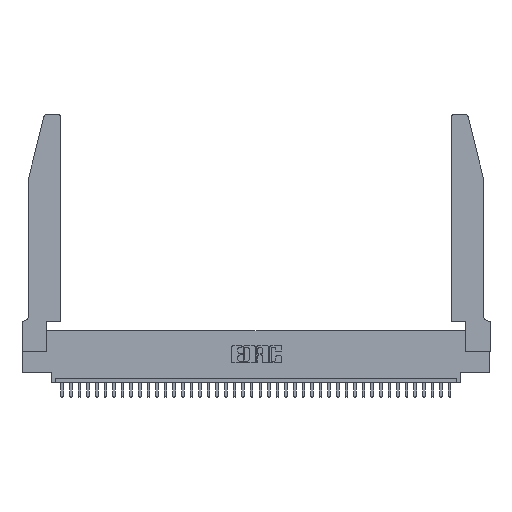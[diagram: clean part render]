
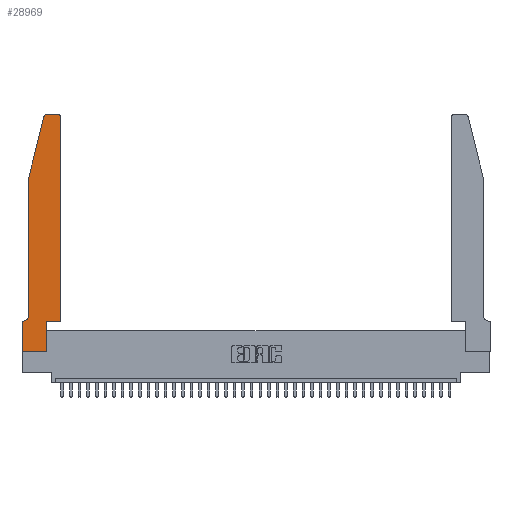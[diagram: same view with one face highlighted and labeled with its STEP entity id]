
A CAD part, top view. The second image highlights one B-rep face of the part: STEP entity #28969.
In plain terms, the highlighted planar face has unit normal (0, 0, 1).
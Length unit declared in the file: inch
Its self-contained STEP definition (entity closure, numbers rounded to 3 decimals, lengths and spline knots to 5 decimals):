
#128 = LINE ( 'NONE', #25591, #30312 ) ;
#791 = CARTESIAN_POINT ( 'NONE',  ( 0.4505, 0.35, 0.37 ) ) ;
#982 = CARTESIAN_POINT ( 'NONE',  ( 0.4505, 0.35, 0.37 ) ) ;
#1350 = VECTOR ( 'NONE', #25044, 39.37008 ) ;
#1521 = VERTEX_POINT ( 'NONE', #6989 ) ;
#1941 = CARTESIAN_POINT ( 'NONE',  ( 0., 0.35, 0.37 ) ) ;
#2319 = LINE ( 'NONE', #22248, #1350 ) ;
#2846 = EDGE_CURVE ( 'NONE', #31651, #19079, #12130, .T. ) ;
#3792 = DIRECTION ( 'NONE',  ( -1., 0., 0. ) ) ;
#3812 = DIRECTION ( 'NONE',  ( 1., 0., 0. ) ) ;
#4138 = DIRECTION ( 'NONE',  ( 0., 0., 1. ) ) ;
#4660 = DIRECTION ( 'NONE',  ( 1., 0., 0. ) ) ;
#4921 = ORIENTED_EDGE ( 'NONE', *, *, #25718, .T. ) ;
#4977 = VERTEX_POINT ( 'NONE', #23273 ) ;
#5688 = VECTOR ( 'NONE', #35818, 39.37008 ) ;
#5738 = VERTEX_POINT ( 'NONE', #27269 ) ;
#5854 = DIRECTION ( 'NONE',  ( 0., -1., 0. ) ) ;
#6151 = EDGE_CURVE ( 'NONE', #10731, #8909, #2319, .T. ) ;
#6451 = VERTEX_POINT ( 'NONE', #10563 ) ;
#6634 = ORIENTED_EDGE ( 'NONE', *, *, #23860, .T. ) ;
#6649 = LINE ( 'NONE', #34305, #27004 ) ;
#6671 = EDGE_LOOP ( 'NONE', ( #28774, #6634, #18262, #8456, #10454, #37717, #17389, #11068, #31452, #4921, #36586, #11282 ) ) ;
#6717 = VECTOR ( 'NONE', #5854, 39.37008 ) ;
#6989 = CARTESIAN_POINT ( 'NONE',  ( 0.2865, 0., 0.37 ) ) ;
#7357 = VERTEX_POINT ( 'NONE', #791 ) ;
#7821 = AXIS2_PLACEMENT_3D ( 'NONE', #34292, #33864, #3812 ) ;
#7995 = PLANE ( 'NONE',  #35997 ) ;
#8456 = ORIENTED_EDGE ( 'NONE', *, *, #28967, .T. ) ;
#8909 = VERTEX_POINT ( 'NONE', #16999 ) ;
#9334 = CARTESIAN_POINT ( 'NONE',  ( 0.2865, 0.35, 0.37 ) ) ;
#9813 = DIRECTION ( 'NONE',  ( 0., 0., -1. ) ) ;
#10454 = ORIENTED_EDGE ( 'NONE', *, *, #38095, .T. ) ;
#10563 = CARTESIAN_POINT ( 'NONE',  ( 0.25487, 2.72718, 0.37 ) ) ;
#10731 = VERTEX_POINT ( 'NONE', #34325 ) ;
#11068 = ORIENTED_EDGE ( 'NONE', *, *, #13427, .T. ) ;
#11282 = ORIENTED_EDGE ( 'NONE', *, *, #33026, .T. ) ;
#11543 = DIRECTION ( 'NONE',  ( 1., 0., 0. ) ) ;
#11690 = CARTESIAN_POINT ( 'NONE',  ( 0.0755, 2., 0.37 ) ) ;
#11742 = LINE ( 'NONE', #982, #18739 ) ;
#11847 = LINE ( 'NONE', #9334, #31189 ) ;
#12130 = LINE ( 'NONE', #37443, #17319 ) ;
#13427 = EDGE_CURVE ( 'NONE', #4977, #1521, #6649, .T. ) ;
#14121 = EDGE_CURVE ( 'NONE', #1521, #28486, #11847, .T. ) ;
#14594 = FACE_OUTER_BOUND ( 'NONE', #6671, .T. ) ;
#15900 = DIRECTION ( 'NONE',  ( -1., 0., 0. ) ) ;
#15913 = EDGE_CURVE ( 'NONE', #7357, #5738, #11742, .T. ) ;
#16732 = DIRECTION ( 'NONE',  ( 1., 0., 0. ) ) ;
#16999 = CARTESIAN_POINT ( 'NONE',  ( 0., 0.35, 0.37 ) ) ;
#17319 = VECTOR ( 'NONE', #3792, 39.37008 ) ;
#17389 = ORIENTED_EDGE ( 'NONE', *, *, #32814, .T. ) ;
#17987 = CIRCLE ( 'NONE', #26717, 0.03 ) ;
#18262 = ORIENTED_EDGE ( 'NONE', *, *, #22320, .T. ) ;
#18739 = VECTOR ( 'NONE', #24847, 39.37008 ) ;
#19079 = VERTEX_POINT ( 'NONE', #31650 ) ;
#19757 = AXIS2_PLACEMENT_3D ( 'NONE', #37557, #9813, #15900 ) ;
#19985 = DIRECTION ( 'NONE',  ( 0., -1., 0. ) ) ;
#21511 = CARTESIAN_POINT ( 'NONE',  ( 0., 0., 0.37 ) ) ;
#22248 = CARTESIAN_POINT ( 'NONE',  ( 0.0755, 0.35, 0.37 ) ) ;
#22320 = EDGE_CURVE ( 'NONE', #6451, #22796, #26927, .T. ) ;
#22796 = VERTEX_POINT ( 'NONE', #31277 ) ;
#23273 = CARTESIAN_POINT ( 'NONE',  ( 0., 0., 0.37 ) ) ;
#23291 = LINE ( 'NONE', #21511, #6717 ) ;
#23860 = EDGE_CURVE ( 'NONE', #19079, #6451, #23974, .T. ) ;
#23974 = CIRCLE ( 'NONE', #7821, 0.03 ) ;
#24756 = CARTESIAN_POINT ( 'NONE',  ( 0.2865, 0.35, 0.37 ) ) ;
#24847 = DIRECTION ( 'NONE',  ( 0., 1., 0. ) ) ;
#25044 = DIRECTION ( 'NONE',  ( -1., 0., 0. ) ) ;
#25152 = VERTEX_POINT ( 'NONE', #37725 ) ;
#25591 = CARTESIAN_POINT ( 'NONE',  ( 0.4505, 0.35, 0.37 ) ) ;
#25718 = EDGE_CURVE ( 'NONE', #28486, #7357, #128, .T. ) ;
#26717 = AXIS2_PLACEMENT_3D ( 'NONE', #37647, #4138, #37366 ) ;
#26855 = LINE ( 'NONE', #34243, #36708 ) ;
#26927 = LINE ( 'NONE', #11690, #5688 ) ;
#27004 = VECTOR ( 'NONE', #4660, 39.37008 ) ;
#27269 = CARTESIAN_POINT ( 'NONE',  ( 0.4505, 2.72, 0.37 ) ) ;
#28486 = VERTEX_POINT ( 'NONE', #24756 ) ;
#28774 = ORIENTED_EDGE ( 'NONE', *, *, #2846, .T. ) ;
#28967 = EDGE_CURVE ( 'NONE', #22796, #25152, #26855, .T. ) ;
#28969 = ADVANCED_FACE ( 'NONE', ( #14594 ), #7995, .T. ) ;
#29035 = CIRCLE ( 'NONE', #19757, 0.07 ) ;
#30312 = VECTOR ( 'NONE', #16732, 39.37008 ) ;
#31137 = DIRECTION ( 'NONE',  ( 0., 1., 0. ) ) ;
#31189 = VECTOR ( 'NONE', #31137, 39.37008 ) ;
#31277 = CARTESIAN_POINT ( 'NONE',  ( 0.0755, 2., 0.37 ) ) ;
#31452 = ORIENTED_EDGE ( 'NONE', *, *, #14121, .T. ) ;
#31650 = CARTESIAN_POINT ( 'NONE',  ( 0.284, 2.75, 0.37 ) ) ;
#31651 = VERTEX_POINT ( 'NONE', #36376 ) ;
#32814 = EDGE_CURVE ( 'NONE', #8909, #4977, #23291, .T. ) ;
#33026 = EDGE_CURVE ( 'NONE', #5738, #31651, #17987, .T. ) ;
#33864 = DIRECTION ( 'NONE',  ( 0., 0., 1. ) ) ;
#34243 = CARTESIAN_POINT ( 'NONE',  ( 0.0755, 2., 0.37 ) ) ;
#34292 = CARTESIAN_POINT ( 'NONE',  ( 0.284, 2.72, 0.37 ) ) ;
#34305 = CARTESIAN_POINT ( 'NONE',  ( 0., 0., 0.37 ) ) ;
#34325 = CARTESIAN_POINT ( 'NONE',  ( 0.0055, 0.35, 0.37 ) ) ;
#35818 = DIRECTION ( 'NONE',  ( -0.239, -0.971, 0. ) ) ;
#35997 = AXIS2_PLACEMENT_3D ( 'NONE', #1941, #38864, #11543 ) ;
#36376 = CARTESIAN_POINT ( 'NONE',  ( 0.4205, 2.75, 0.37 ) ) ;
#36586 = ORIENTED_EDGE ( 'NONE', *, *, #15913, .T. ) ;
#36708 = VECTOR ( 'NONE', #19985, 39.37008 ) ;
#37366 = DIRECTION ( 'NONE',  ( 1., 0., 0. ) ) ;
#37443 = CARTESIAN_POINT ( 'NONE',  ( 0.2605, 2.75, 0.37 ) ) ;
#37557 = CARTESIAN_POINT ( 'NONE',  ( 0.0055, 0.42, 0.37 ) ) ;
#37647 = CARTESIAN_POINT ( 'NONE',  ( 0.4205, 2.72, 0.37 ) ) ;
#37717 = ORIENTED_EDGE ( 'NONE', *, *, #6151, .T. ) ;
#37725 = CARTESIAN_POINT ( 'NONE',  ( 0.0755, 0.42, 0.37 ) ) ;
#38095 = EDGE_CURVE ( 'NONE', #25152, #10731, #29035, .T. ) ;
#38864 = DIRECTION ( 'NONE',  ( 0., 0., 1. ) ) ;
